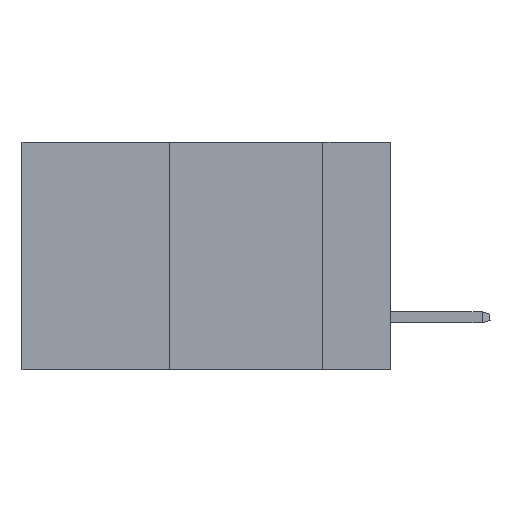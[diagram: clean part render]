
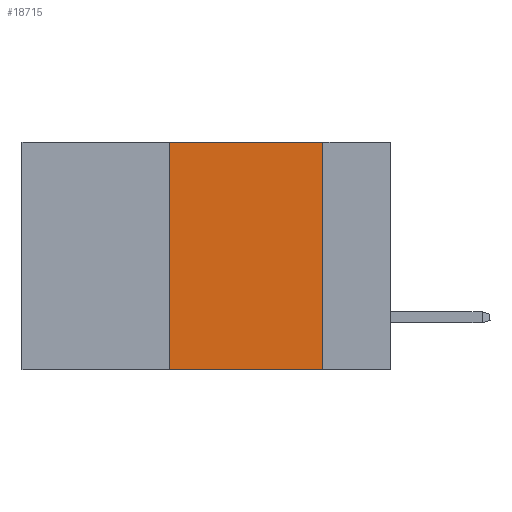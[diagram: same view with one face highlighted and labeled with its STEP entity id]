
A CAD part, left-side view. The second image highlights one B-rep face of the part: STEP entity #18715.
In plain terms, the highlighted planar face has unit normal (-1, 0, 0).
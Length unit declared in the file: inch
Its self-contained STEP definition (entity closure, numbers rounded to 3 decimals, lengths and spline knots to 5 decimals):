
#1972 = VERTEX_POINT ( 'NONE', #5635 ) ;
#2752 = CARTESIAN_POINT ( 'NONE',  ( 0., 0.11, 0. ) ) ;
#3184 = ORIENTED_EDGE ( 'NONE', *, *, #7016, .T. ) ;
#3438 = VERTEX_POINT ( 'NONE', #7163 ) ;
#4513 = ORIENTED_EDGE ( 'NONE', *, *, #5111, .F. ) ;
#4881 = EDGE_LOOP ( 'NONE', ( #6379, #4513, #10400, #3184 ) ) ;
#5090 = VECTOR ( 'NONE', #18390, 39.37008 ) ;
#5111 = EDGE_CURVE ( 'NONE', #15460, #3438, #13625, .T. ) ;
#5263 = LINE ( 'NONE', #5295, #11381 ) ;
#5295 = CARTESIAN_POINT ( 'NONE',  ( 0., 0.6, -0.37 ) ) ;
#5635 = CARTESIAN_POINT ( 'NONE',  ( 0., 0.36, -0.37 ) ) ;
#6379 = ORIENTED_EDGE ( 'NONE', *, *, #10544, .F. ) ;
#6920 = CARTESIAN_POINT ( 'NONE',  ( 0., 0.36, 0. ) ) ;
#7016 = EDGE_CURVE ( 'NONE', #1972, #8756, #5263, .T. ) ;
#7163 = CARTESIAN_POINT ( 'NONE',  ( 0., 0.11, 0. ) ) ;
#7820 = CARTESIAN_POINT ( 'NONE',  ( 0., 0.6, 0. ) ) ;
#7891 = DIRECTION ( 'NONE',  ( 0., 0., -1. ) ) ;
#8756 = VERTEX_POINT ( 'NONE', #21052 ) ;
#9156 = LINE ( 'NONE', #2752, #16557 ) ;
#10400 = ORIENTED_EDGE ( 'NONE', *, *, #18351, .F. ) ;
#10415 = DIRECTION ( 'NONE',  ( 0., -1., 0. ) ) ;
#10544 = EDGE_CURVE ( 'NONE', #3438, #8756, #9156, .T. ) ;
#11381 = VECTOR ( 'NONE', #10415, 39.37008 ) ;
#12562 = CARTESIAN_POINT ( 'NONE',  ( 0., 0.36, 0. ) ) ;
#13063 = LINE ( 'NONE', #12562, #21260 ) ;
#13577 = CARTESIAN_POINT ( 'NONE',  ( 0., 0.6, 0. ) ) ;
#13625 = LINE ( 'NONE', #13577, #5090 ) ;
#14274 = DIRECTION ( 'NONE',  ( 0., 0., 1. ) ) ;
#14501 = AXIS2_PLACEMENT_3D ( 'NONE', #7820, #21339, #7891 ) ;
#14562 = DIRECTION ( 'NONE',  ( 0., 0., -1. ) ) ;
#14912 = FACE_OUTER_BOUND ( 'NONE', #4881, .T. ) ;
#15460 = VERTEX_POINT ( 'NONE', #6920 ) ;
#16557 = VECTOR ( 'NONE', #14562, 39.37008 ) ;
#18351 = EDGE_CURVE ( 'NONE', #1972, #15460, #13063, .T. ) ;
#18390 = DIRECTION ( 'NONE',  ( 0., -1., 0. ) ) ;
#18715 = ADVANCED_FACE ( 'NONE', ( #14912 ), #19538, .F. ) ;
#19538 = PLANE ( 'NONE',  #14501 ) ;
#21052 = CARTESIAN_POINT ( 'NONE',  ( 0., 0.11, -0.37 ) ) ;
#21260 = VECTOR ( 'NONE', #14274, 39.37008 ) ;
#21339 = DIRECTION ( 'NONE',  ( 1., 0., 0. ) ) ;
